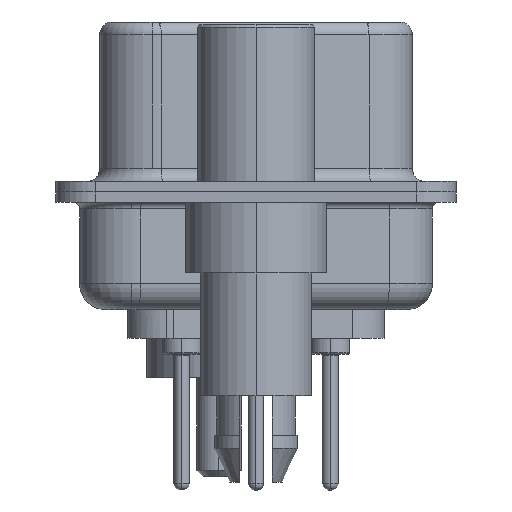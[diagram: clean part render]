
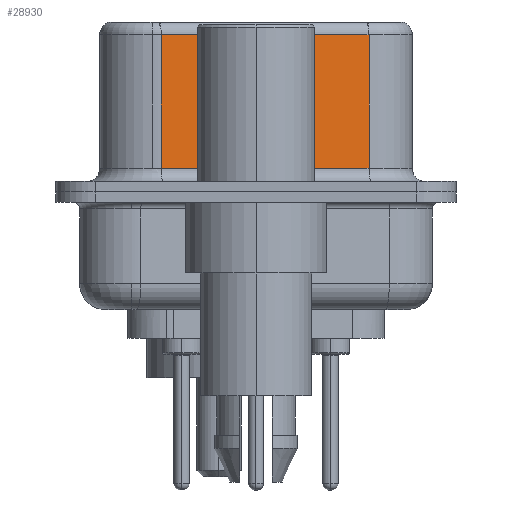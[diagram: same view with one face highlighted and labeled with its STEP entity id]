
A CAD part, left-side view. The second image highlights one B-rep face of the part: STEP entity #28930.
In plain terms, the highlighted planar face has unit normal (-0.985, -0.174, 0).
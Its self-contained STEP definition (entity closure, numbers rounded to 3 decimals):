
#2283 = EDGE_CURVE ( 'NONE', #12660, #23574, #21936, .T. ) ;
#5418 = LINE ( 'NONE', #19630, #31711 ) ;
#6244 = EDGE_CURVE ( 'NONE', #17348, #23148, #28398, .T. ) ;
#7312 = DIRECTION ( 'NONE',  ( 0.174, -0.985, 0. ) ) ;
#8113 = VECTOR ( 'NONE', #32010, 1000. ) ;
#9212 = VECTOR ( 'NONE', #7312, 1000. ) ;
#10426 = CARTESIAN_POINT ( 'NONE',  ( 5.132, -4.322, 6.02 ) ) ;
#12068 = DIRECTION ( 'NONE',  ( 0., 0., -1. ) ) ;
#12660 = VERTEX_POINT ( 'NONE', #22839 ) ;
#13652 = EDGE_CURVE ( 'NONE', #23148, #12660, #14398, .T. ) ;
#13844 = ORIENTED_EDGE ( 'NONE', *, *, #6244, .T. ) ;
#14199 = CARTESIAN_POINT ( 'NONE',  ( 5.132, -4.322, 6.02 ) ) ;
#14398 = LINE ( 'NONE', #19989, #27908 ) ;
#16910 = FACE_OUTER_BOUND ( 'NONE', #21568, .T. ) ;
#17035 = DIRECTION ( 'NONE',  ( -0.174, 0.985, 0. ) ) ;
#17348 = VERTEX_POINT ( 'NONE', #10426 ) ;
#18581 = AXIS2_PLACEMENT_3D ( 'NONE', #29569, #32277, #17035 ) ;
#19114 = EDGE_CURVE ( 'NONE', #17348, #23574, #5418, .T. ) ;
#19630 = CARTESIAN_POINT ( 'NONE',  ( 5.132, -4.322, 6.52 ) ) ;
#19989 = CARTESIAN_POINT ( 'NONE',  ( 3.73, 3.628, 6.52 ) ) ;
#21568 = EDGE_LOOP ( 'NONE', ( #27540, #13844, #26746, #23942 ) ) ;
#21936 = LINE ( 'NONE', #31566, #9212 ) ;
#22538 = DIRECTION ( 'NONE',  ( 0., 0., -1. ) ) ;
#22839 = CARTESIAN_POINT ( 'NONE',  ( 3.73, 3.628, 0.9 ) ) ;
#23148 = VERTEX_POINT ( 'NONE', #32832 ) ;
#23574 = VERTEX_POINT ( 'NONE', #26947 ) ;
#23942 = ORIENTED_EDGE ( 'NONE', *, *, #2283, .T. ) ;
#26746 = ORIENTED_EDGE ( 'NONE', *, *, #13652, .T. ) ;
#26947 = CARTESIAN_POINT ( 'NONE',  ( 5.132, -4.322, 0.9 ) ) ;
#27540 = ORIENTED_EDGE ( 'NONE', *, *, #19114, .F. ) ;
#27908 = VECTOR ( 'NONE', #22538, 1000. ) ;
#28398 = LINE ( 'NONE', #14199, #8113 ) ;
#28930 = ADVANCED_FACE ( 'NONE', ( #16910 ), #29672, .F. ) ;
#29569 = CARTESIAN_POINT ( 'NONE',  ( 5.132, -4.322, 6.52 ) ) ;
#29672 = PLANE ( 'NONE',  #18581 ) ;
#31566 = CARTESIAN_POINT ( 'NONE',  ( 5.132, -4.322, 0.9 ) ) ;
#31711 = VECTOR ( 'NONE', #12068, 1000. ) ;
#32010 = DIRECTION ( 'NONE',  ( -0.174, 0.985, 0. ) ) ;
#32277 = DIRECTION ( 'NONE',  ( 0.985, 0.174, 0. ) ) ;
#32832 = CARTESIAN_POINT ( 'NONE',  ( 3.73, 3.628, 6.02 ) ) ;
